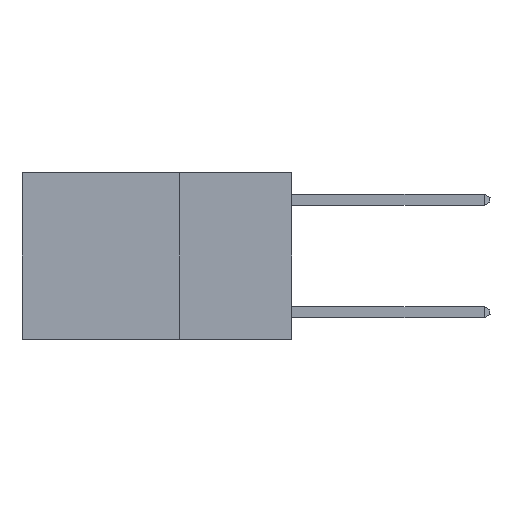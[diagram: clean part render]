
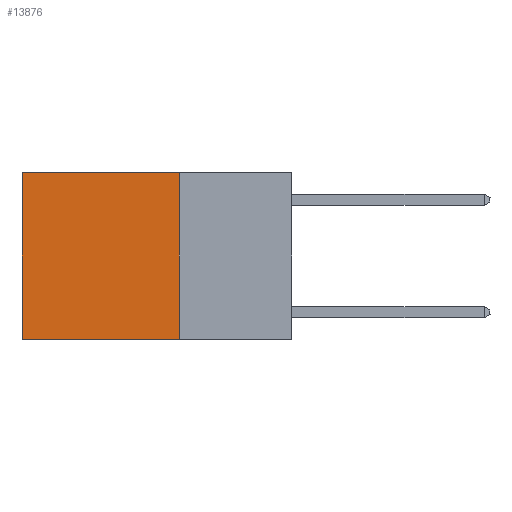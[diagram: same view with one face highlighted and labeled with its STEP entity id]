
A CAD part, left-side view. The second image highlights one B-rep face of the part: STEP entity #13876.
In plain terms, the highlighted planar face has unit normal (-1, 0, 0).
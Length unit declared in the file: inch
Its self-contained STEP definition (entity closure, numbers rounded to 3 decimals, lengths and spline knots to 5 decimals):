
#1329 = DIRECTION ( 'NONE',  ( 0., 1., 0. ) ) ;
#2225 = EDGE_LOOP ( 'NONE', ( #8347, #19185, #7180, #9968 ) ) ;
#3463 = DIRECTION ( 'NONE',  ( 0., 0., -1. ) ) ;
#4620 = DIRECTION ( 'NONE',  ( 0., 1., 0. ) ) ;
#6324 = CARTESIAN_POINT ( 'NONE',  ( 0.2625, 0.25, 0. ) ) ;
#6655 = CARTESIAN_POINT ( 'NONE',  ( 0.2625, 0.25, 0. ) ) ;
#7011 = CARTESIAN_POINT ( 'NONE',  ( 0.2625, 0.6, 0. ) ) ;
#7180 = ORIENTED_EDGE ( 'NONE', *, *, #11835, .F. ) ;
#7799 = CARTESIAN_POINT ( 'NONE',  ( 0.2625, 0.25, -0.37 ) ) ;
#8347 = ORIENTED_EDGE ( 'NONE', *, *, #10576, .T. ) ;
#8806 = VECTOR ( 'NONE', #1329, 39.37008 ) ;
#8908 = VECTOR ( 'NONE', #4620, 39.37008 ) ;
#9968 = ORIENTED_EDGE ( 'NONE', *, *, #10552, .T. ) ;
#10331 = DIRECTION ( 'NONE',  ( 0., 0., -1. ) ) ;
#10552 = EDGE_CURVE ( 'NONE', #12396, #11199, #10987, .T. ) ;
#10576 = EDGE_CURVE ( 'NONE', #11199, #17387, #18957, .T. ) ;
#10987 = LINE ( 'NONE', #17135, #8908 ) ;
#11004 = VECTOR ( 'NONE', #17137, 39.37008 ) ;
#11199 = VERTEX_POINT ( 'NONE', #7011 ) ;
#11250 = PLANE ( 'NONE',  #18437 ) ;
#11350 = DIRECTION ( 'NONE',  ( 1., 0., 0. ) ) ;
#11431 = CARTESIAN_POINT ( 'NONE',  ( 0.2625, 0.6, -0.37 ) ) ;
#11518 = VECTOR ( 'NONE', #10331, 39.37008 ) ;
#11835 = EDGE_CURVE ( 'NONE', #12396, #19390, #15537, .T. ) ;
#12396 = VERTEX_POINT ( 'NONE', #17721 ) ;
#12548 = EDGE_CURVE ( 'NONE', #19390, #17387, #15299, .T. ) ;
#13876 = ADVANCED_FACE ( 'NONE', ( #18926 ), #11250, .F. ) ;
#15299 = LINE ( 'NONE', #18232, #8806 ) ;
#15437 = CARTESIAN_POINT ( 'NONE',  ( 0.2625, 0.6, 0. ) ) ;
#15537 = LINE ( 'NONE', #6655, #11004 ) ;
#17135 = CARTESIAN_POINT ( 'NONE',  ( 0.2625, 0.25, 0. ) ) ;
#17137 = DIRECTION ( 'NONE',  ( 0., 0., -1. ) ) ;
#17387 = VERTEX_POINT ( 'NONE', #11431 ) ;
#17721 = CARTESIAN_POINT ( 'NONE',  ( 0.2625, 0.25, 0. ) ) ;
#18232 = CARTESIAN_POINT ( 'NONE',  ( 0.2625, 0.25, -0.37 ) ) ;
#18437 = AXIS2_PLACEMENT_3D ( 'NONE', #6324, #11350, #3463 ) ;
#18926 = FACE_OUTER_BOUND ( 'NONE', #2225, .T. ) ;
#18957 = LINE ( 'NONE', #15437, #11518 ) ;
#19185 = ORIENTED_EDGE ( 'NONE', *, *, #12548, .F. ) ;
#19390 = VERTEX_POINT ( 'NONE', #7799 ) ;
